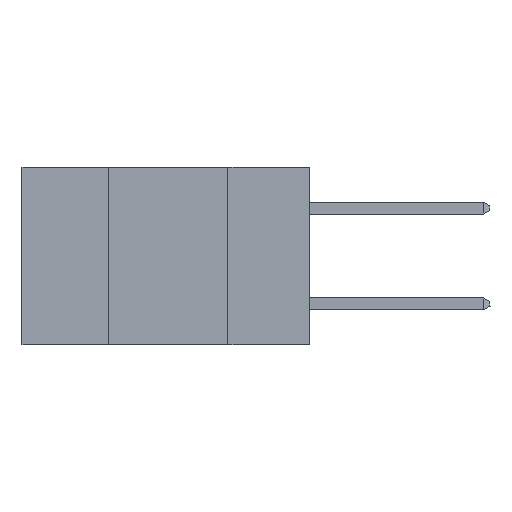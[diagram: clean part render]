
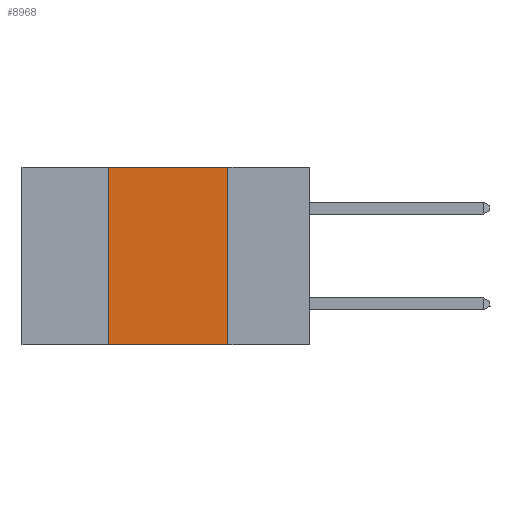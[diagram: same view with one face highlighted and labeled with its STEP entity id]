
A CAD part, left-side view. The second image highlights one B-rep face of the part: STEP entity #8968.
In plain terms, the highlighted planar face has unit normal (-1, 0, 0).
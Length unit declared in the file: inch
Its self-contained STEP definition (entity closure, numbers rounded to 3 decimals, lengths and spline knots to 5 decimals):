
#379 = EDGE_LOOP ( 'NONE', ( #2199, #8466, #1665, #2412 ) ) ;
#739 = VERTEX_POINT ( 'NONE', #10054 ) ;
#1346 = CARTESIAN_POINT ( 'NONE',  ( 0., 0.6, -0.37 ) ) ;
#1665 = ORIENTED_EDGE ( 'NONE', *, *, #4141, .F. ) ;
#2199 = ORIENTED_EDGE ( 'NONE', *, *, #8836, .F. ) ;
#2374 = VECTOR ( 'NONE', #3200, 39.37008 ) ;
#2381 = CARTESIAN_POINT ( 'NONE',  ( 0., 0.6, 0. ) ) ;
#2385 = LINE ( 'NONE', #8194, #6170 ) ;
#2412 = ORIENTED_EDGE ( 'NONE', *, *, #2492, .T. ) ;
#2489 = VERTEX_POINT ( 'NONE', #9200 ) ;
#2492 = EDGE_CURVE ( 'NONE', #6392, #3379, #10251, .T. ) ;
#2994 = CARTESIAN_POINT ( 'NONE',  ( 0., 0.6, 0. ) ) ;
#3019 = LINE ( 'NONE', #3537, #9027 ) ;
#3200 = DIRECTION ( 'NONE',  ( 0., -1., 0. ) ) ;
#3379 = VERTEX_POINT ( 'NONE', #8843 ) ;
#3537 = CARTESIAN_POINT ( 'NONE',  ( 0., 0.17, 0. ) ) ;
#3831 = DIRECTION ( 'NONE',  ( 1., 0., 0. ) ) ;
#4141 = EDGE_CURVE ( 'NONE', #6392, #2489, #2385, .T. ) ;
#4167 = FACE_OUTER_BOUND ( 'NONE', #379, .T. ) ;
#4354 = DIRECTION ( 'NONE',  ( 0., 0., -1. ) ) ;
#4547 = EDGE_CURVE ( 'NONE', #2489, #739, #6641, .T. ) ;
#6170 = VECTOR ( 'NONE', #8996, 39.37008 ) ;
#6274 = CARTESIAN_POINT ( 'NONE',  ( 0., 0.42, -0.37 ) ) ;
#6392 = VERTEX_POINT ( 'NONE', #6274 ) ;
#6641 = LINE ( 'NONE', #2381, #2374 ) ;
#8120 = AXIS2_PLACEMENT_3D ( 'NONE', #2994, #3831, #9276 ) ;
#8194 = CARTESIAN_POINT ( 'NONE',  ( 0., 0.42, 0. ) ) ;
#8452 = VECTOR ( 'NONE', #8457, 39.37008 ) ;
#8457 = DIRECTION ( 'NONE',  ( 0., -1., 0. ) ) ;
#8466 = ORIENTED_EDGE ( 'NONE', *, *, #4547, .F. ) ;
#8496 = PLANE ( 'NONE',  #8120 ) ;
#8836 = EDGE_CURVE ( 'NONE', #739, #3379, #3019, .T. ) ;
#8843 = CARTESIAN_POINT ( 'NONE',  ( 0., 0.17, -0.37 ) ) ;
#8968 = ADVANCED_FACE ( 'NONE', ( #4167 ), #8496, .F. ) ;
#8996 = DIRECTION ( 'NONE',  ( 0., 0., 1. ) ) ;
#9027 = VECTOR ( 'NONE', #4354, 39.37008 ) ;
#9200 = CARTESIAN_POINT ( 'NONE',  ( 0., 0.42, 0. ) ) ;
#9276 = DIRECTION ( 'NONE',  ( 0., 0., -1. ) ) ;
#10054 = CARTESIAN_POINT ( 'NONE',  ( 0., 0.17, 0. ) ) ;
#10251 = LINE ( 'NONE', #1346, #8452 ) ;
